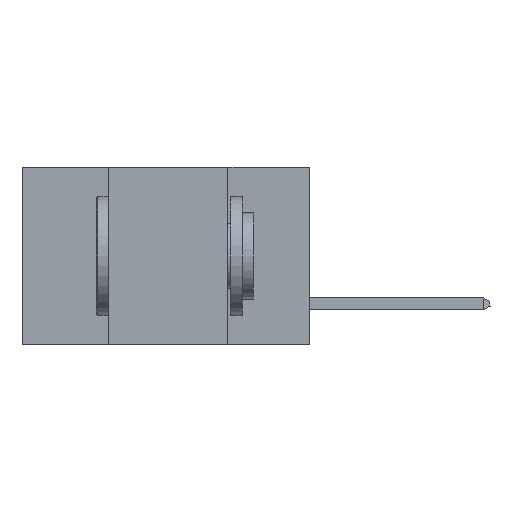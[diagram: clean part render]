
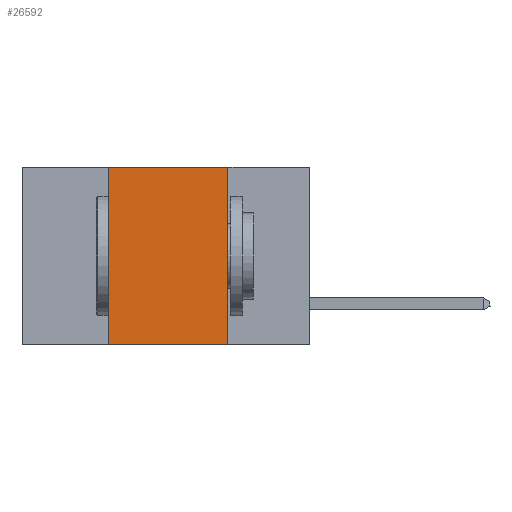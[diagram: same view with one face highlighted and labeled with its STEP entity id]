
A CAD part, left-side view. The second image highlights one B-rep face of the part: STEP entity #26592.
In plain terms, the highlighted planar face has unit normal (-1, 0, 0).
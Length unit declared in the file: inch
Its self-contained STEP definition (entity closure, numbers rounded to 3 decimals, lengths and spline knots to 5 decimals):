
#13 = DIRECTION ( 'NONE',  ( 0., -1., 0. ) ) ;
#1202 = ORIENTED_EDGE ( 'NONE', *, *, #25008, .T. ) ;
#2327 = VERTEX_POINT ( 'NONE', #17328 ) ;
#2658 = CARTESIAN_POINT ( 'NONE',  ( 0., 0.42, 0. ) ) ;
#2759 = LINE ( 'NONE', #8918, #11425 ) ;
#2764 = DIRECTION ( 'NONE',  ( 0., 0., 1. ) ) ;
#2937 = DIRECTION ( 'NONE',  ( 0., -1., 0. ) ) ;
#4799 = PLANE ( 'NONE',  #17850 ) ;
#5308 = VECTOR ( 'NONE', #13, 39.37008 ) ;
#6440 = VERTEX_POINT ( 'NONE', #14097 ) ;
#7141 = VECTOR ( 'NONE', #15322, 39.37008 ) ;
#8918 = CARTESIAN_POINT ( 'NONE',  ( 0., 0.42, 0. ) ) ;
#9177 = DIRECTION ( 'NONE',  ( 0., 0., -1. ) ) ;
#10252 = FACE_OUTER_BOUND ( 'NONE', #26712, .T. ) ;
#10484 = CARTESIAN_POINT ( 'NONE',  ( 0., 0.42, -0.37 ) ) ;
#11425 = VECTOR ( 'NONE', #2764, 39.37008 ) ;
#11913 = CARTESIAN_POINT ( 'NONE',  ( 0., 0.17, 0. ) ) ;
#14097 = CARTESIAN_POINT ( 'NONE',  ( 0., 0.17, 0. ) ) ;
#14953 = ORIENTED_EDGE ( 'NONE', *, *, #17159, .F. ) ;
#15322 = DIRECTION ( 'NONE',  ( 0., 0., -1. ) ) ;
#15741 = EDGE_CURVE ( 'NONE', #6440, #2327, #25415, .T. ) ;
#16031 = ORIENTED_EDGE ( 'NONE', *, *, #23364, .F. ) ;
#17159 = EDGE_CURVE ( 'NONE', #26892, #6440, #21441, .T. ) ;
#17328 = CARTESIAN_POINT ( 'NONE',  ( 0., 0.17, -0.37 ) ) ;
#17850 = AXIS2_PLACEMENT_3D ( 'NONE', #17997, #17905, #9177 ) ;
#17905 = DIRECTION ( 'NONE',  ( 1., 0., 0. ) ) ;
#17997 = CARTESIAN_POINT ( 'NONE',  ( 0., 0.6, 0. ) ) ;
#19771 = CARTESIAN_POINT ( 'NONE',  ( 0., 0.6, 0. ) ) ;
#20629 = LINE ( 'NONE', #26976, #5308 ) ;
#21441 = LINE ( 'NONE', #19771, #25046 ) ;
#22768 = ORIENTED_EDGE ( 'NONE', *, *, #15741, .F. ) ;
#23364 = EDGE_CURVE ( 'NONE', #26943, #26892, #2759, .T. ) ;
#25008 = EDGE_CURVE ( 'NONE', #26943, #2327, #20629, .T. ) ;
#25046 = VECTOR ( 'NONE', #2937, 39.37008 ) ;
#25415 = LINE ( 'NONE', #11913, #7141 ) ;
#26592 = ADVANCED_FACE ( 'NONE', ( #10252 ), #4799, .F. ) ;
#26712 = EDGE_LOOP ( 'NONE', ( #22768, #14953, #16031, #1202 ) ) ;
#26892 = VERTEX_POINT ( 'NONE', #2658 ) ;
#26943 = VERTEX_POINT ( 'NONE', #10484 ) ;
#26976 = CARTESIAN_POINT ( 'NONE',  ( 0., 0.6, -0.37 ) ) ;
